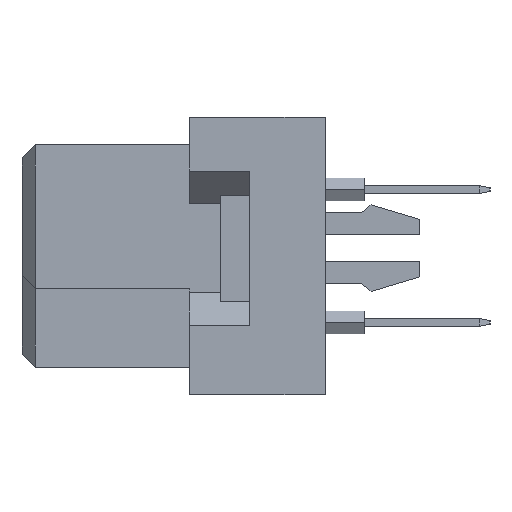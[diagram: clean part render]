
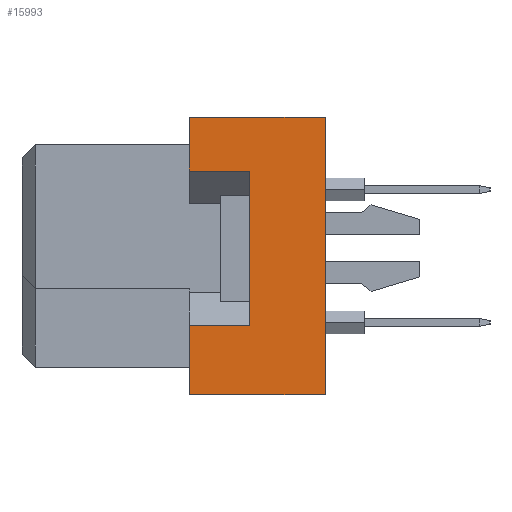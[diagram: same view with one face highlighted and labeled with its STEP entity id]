
A CAD part, left-side view. The second image highlights one B-rep face of the part: STEP entity #15993.
In plain terms, the highlighted planar face has unit normal (-1, 0, 0).
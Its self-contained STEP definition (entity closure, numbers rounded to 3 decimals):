
#154 = EDGE_CURVE ( 'NONE', #12056, #15359, #10536, .T. ) ;
#167 = ORIENTED_EDGE ( 'NONE', *, *, #154, .T. ) ;
#546 = CARTESIAN_POINT ( 'NONE',  ( -47.5, -11.6, 5.3 ) ) ;
#2059 = VECTOR ( 'NONE', #20430, 1000. ) ;
#2596 = CARTESIAN_POINT ( 'NONE',  ( -47.5, -8.7, -2.65 ) ) ;
#3373 = EDGE_LOOP ( 'NONE', ( #8591, #18546, #31206, #21271, #167, #32488, #29645, #25552 ) ) ;
#3377 = CARTESIAN_POINT ( 'NONE',  ( -47.5, -11.6, -5.3 ) ) ;
#3503 = LINE ( 'NONE', #40353, #7281 ) ;
#4153 = CARTESIAN_POINT ( 'NONE',  ( -47.5, -11.6, 5.3 ) ) ;
#4476 = LINE ( 'NONE', #19321, #19166 ) ;
#4768 = EDGE_CURVE ( 'NONE', #5500, #25965, #12283, .T. ) ;
#5500 = VERTEX_POINT ( 'NONE', #23511 ) ;
#5564 = EDGE_CURVE ( 'NONE', #5500, #39863, #35647, .T. ) ;
#5709 = VECTOR ( 'NONE', #37660, 1000. ) ;
#5975 = CARTESIAN_POINT ( 'NONE',  ( -47.5, -6.4, -5.3 ) ) ;
#7131 = AXIS2_PLACEMENT_3D ( 'NONE', #16756, #10571, #23125 ) ;
#7281 = VECTOR ( 'NONE', #12585, 1000. ) ;
#8591 = ORIENTED_EDGE ( 'NONE', *, *, #5564, .T. ) ;
#9927 = VERTEX_POINT ( 'NONE', #36876 ) ;
#10536 = LINE ( 'NONE', #4153, #11897 ) ;
#10571 = DIRECTION ( 'NONE',  ( -1., 0., 0. ) ) ;
#10819 = CARTESIAN_POINT ( 'NONE',  ( -47.5, -8.7, 3.25 ) ) ;
#11872 = CARTESIAN_POINT ( 'NONE',  ( -47.5, -6.4, -5.3 ) ) ;
#11897 = VECTOR ( 'NONE', #35418, 1000. ) ;
#12056 = VERTEX_POINT ( 'NONE', #546 ) ;
#12283 = LINE ( 'NONE', #2596, #39652 ) ;
#12346 = CARTESIAN_POINT ( 'NONE',  ( -47.5, -6.4, 5.3 ) ) ;
#12585 = DIRECTION ( 'NONE',  ( 0., 0., 1. ) ) ;
#12829 = CARTESIAN_POINT ( 'NONE',  ( -47.5, -6.4, -2.65 ) ) ;
#14706 = CARTESIAN_POINT ( 'NONE',  ( -47.5, -11.6, -5.3 ) ) ;
#15011 = DIRECTION ( 'NONE',  ( 0., 0., 1. ) ) ;
#15265 = LINE ( 'NONE', #5975, #5709 ) ;
#15359 = VERTEX_POINT ( 'NONE', #12346 ) ;
#15993 = ADVANCED_FACE ( 'NONE', ( #22526 ), #28677, .T. ) ;
#16756 = CARTESIAN_POINT ( 'NONE',  ( -47.5, -11.6, 5.3 ) ) ;
#18546 = ORIENTED_EDGE ( 'NONE', *, *, #20584, .F. ) ;
#19166 = VECTOR ( 'NONE', #35349, 1000. ) ;
#19321 = CARTESIAN_POINT ( 'NONE',  ( -47.5, -8.7, 3.25 ) ) ;
#20430 = DIRECTION ( 'NONE',  ( 0., 1., 0. ) ) ;
#20584 = EDGE_CURVE ( 'NONE', #36113, #39863, #3503, .T. ) ;
#21196 = EDGE_CURVE ( 'NONE', #25965, #9927, #4476, .T. ) ;
#21271 = ORIENTED_EDGE ( 'NONE', *, *, #35641, .T. ) ;
#22526 = FACE_OUTER_BOUND ( 'NONE', #3373, .T. ) ;
#23125 = DIRECTION ( 'NONE',  ( 0., 0., 1. ) ) ;
#23139 = VERTEX_POINT ( 'NONE', #3377 ) ;
#23384 = VECTOR ( 'NONE', #15011, 1000. ) ;
#23511 = CARTESIAN_POINT ( 'NONE',  ( -47.5, -8.7, -2.65 ) ) ;
#23753 = LINE ( 'NONE', #14706, #39834 ) ;
#23859 = LINE ( 'NONE', #27758, #23384 ) ;
#24420 = DIRECTION ( 'NONE',  ( 0., 0., 1. ) ) ;
#25552 = ORIENTED_EDGE ( 'NONE', *, *, #4768, .F. ) ;
#25965 = VERTEX_POINT ( 'NONE', #10819 ) ;
#27758 = CARTESIAN_POINT ( 'NONE',  ( -47.5, -11.6, 5.3 ) ) ;
#28677 = PLANE ( 'NONE',  #7131 ) ;
#29645 = ORIENTED_EDGE ( 'NONE', *, *, #21196, .F. ) ;
#31206 = ORIENTED_EDGE ( 'NONE', *, *, #39718, .F. ) ;
#32488 = ORIENTED_EDGE ( 'NONE', *, *, #40589, .F. ) ;
#33616 = DIRECTION ( 'NONE',  ( 0., 1., 0. ) ) ;
#35349 = DIRECTION ( 'NONE',  ( 0., 1., 0. ) ) ;
#35418 = DIRECTION ( 'NONE',  ( 0., 1., 0. ) ) ;
#35641 = EDGE_CURVE ( 'NONE', #23139, #12056, #23859, .T. ) ;
#35647 = LINE ( 'NONE', #36044, #2059 ) ;
#36044 = CARTESIAN_POINT ( 'NONE',  ( -47.5, -8.7, -2.65 ) ) ;
#36113 = VERTEX_POINT ( 'NONE', #11872 ) ;
#36876 = CARTESIAN_POINT ( 'NONE',  ( -47.5, -6.4, 3.25 ) ) ;
#37660 = DIRECTION ( 'NONE',  ( 0., 0., 1. ) ) ;
#39652 = VECTOR ( 'NONE', #24420, 1000. ) ;
#39718 = EDGE_CURVE ( 'NONE', #23139, #36113, #23753, .T. ) ;
#39834 = VECTOR ( 'NONE', #33616, 1000. ) ;
#39863 = VERTEX_POINT ( 'NONE', #12829 ) ;
#40353 = CARTESIAN_POINT ( 'NONE',  ( -47.5, -6.4, -5.3 ) ) ;
#40589 = EDGE_CURVE ( 'NONE', #9927, #15359, #15265, .T. ) ;
